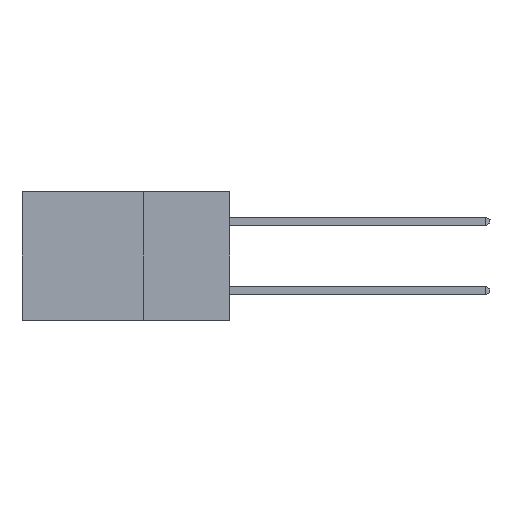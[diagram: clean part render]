
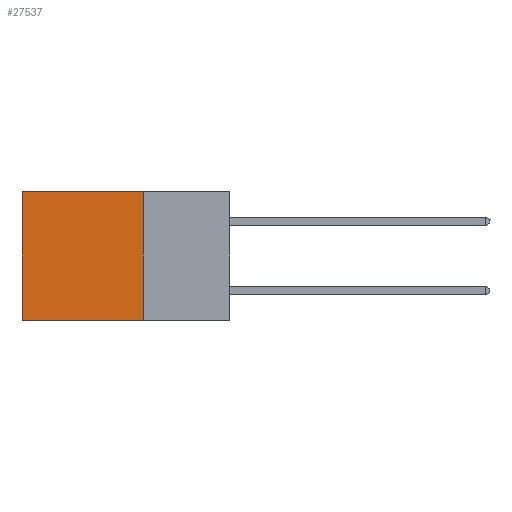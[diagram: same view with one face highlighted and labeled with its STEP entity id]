
A CAD part, left-side view. The second image highlights one B-rep face of the part: STEP entity #27537.
In plain terms, the highlighted planar face has unit normal (-1, 0, 0).
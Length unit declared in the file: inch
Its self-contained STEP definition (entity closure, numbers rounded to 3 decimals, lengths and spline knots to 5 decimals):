
#1925 = ORIENTED_EDGE ( 'NONE', *, *, #22145, .T. ) ;
#2560 = FACE_OUTER_BOUND ( 'NONE', #5401, .T. ) ;
#2870 = VECTOR ( 'NONE', #15265, 39.37008 ) ;
#3825 = DIRECTION ( 'NONE',  ( 0., 0., -1. ) ) ;
#4101 = CARTESIAN_POINT ( 'NONE',  ( 0.298, 0.25, -0.37 ) ) ;
#4138 = DIRECTION ( 'NONE',  ( 0., 1., 0. ) ) ;
#5133 = LINE ( 'NONE', #8567, #9834 ) ;
#5401 = EDGE_LOOP ( 'NONE', ( #16543, #14349, #10480, #1925 ) ) ;
#6050 = CARTESIAN_POINT ( 'NONE',  ( 0.298, 0.25, -0.37 ) ) ;
#6844 = CARTESIAN_POINT ( 'NONE',  ( 0.298, 0.25, 0. ) ) ;
#7336 = CARTESIAN_POINT ( 'NONE',  ( 0.298, 0.6, -0.37 ) ) ;
#8091 = EDGE_CURVE ( 'NONE', #20293, #17822, #8389, .T. ) ;
#8290 = VERTEX_POINT ( 'NONE', #29018 ) ;
#8389 = LINE ( 'NONE', #23202, #15227 ) ;
#8567 = CARTESIAN_POINT ( 'NONE',  ( 0.298, 0.25, 0. ) ) ;
#8704 = CARTESIAN_POINT ( 'NONE',  ( 0.298, 0.6, 0. ) ) ;
#9449 = DIRECTION ( 'NONE',  ( 1., 0., 0. ) ) ;
#9550 = CARTESIAN_POINT ( 'NONE',  ( 0.298, 0.25, 0. ) ) ;
#9834 = VECTOR ( 'NONE', #4138, 39.37008 ) ;
#10260 = EDGE_CURVE ( 'NONE', #21492, #17822, #27780, .T. ) ;
#10480 = ORIENTED_EDGE ( 'NONE', *, *, #16334, .F. ) ;
#11138 = LINE ( 'NONE', #6844, #13316 ) ;
#13316 = VECTOR ( 'NONE', #3825, 39.37008 ) ;
#14349 = ORIENTED_EDGE ( 'NONE', *, *, #10260, .F. ) ;
#15227 = VECTOR ( 'NONE', #18841, 39.37008 ) ;
#15265 = DIRECTION ( 'NONE',  ( 0., 1., 0. ) ) ;
#16334 = EDGE_CURVE ( 'NONE', #8290, #21492, #11138, .T. ) ;
#16543 = ORIENTED_EDGE ( 'NONE', *, *, #8091, .T. ) ;
#17822 = VERTEX_POINT ( 'NONE', #7336 ) ;
#18841 = DIRECTION ( 'NONE',  ( 0., 0., -1. ) ) ;
#20293 = VERTEX_POINT ( 'NONE', #8704 ) ;
#21492 = VERTEX_POINT ( 'NONE', #6050 ) ;
#21660 = AXIS2_PLACEMENT_3D ( 'NONE', #9550, #9449, #23169 ) ;
#22145 = EDGE_CURVE ( 'NONE', #8290, #20293, #5133, .T. ) ;
#23169 = DIRECTION ( 'NONE',  ( 0., 0., -1. ) ) ;
#23202 = CARTESIAN_POINT ( 'NONE',  ( 0.298, 0.6, 0. ) ) ;
#27537 = ADVANCED_FACE ( 'NONE', ( #2560 ), #27698, .F. ) ;
#27698 = PLANE ( 'NONE',  #21660 ) ;
#27780 = LINE ( 'NONE', #4101, #2870 ) ;
#29018 = CARTESIAN_POINT ( 'NONE',  ( 0.298, 0.25, 0. ) ) ;
